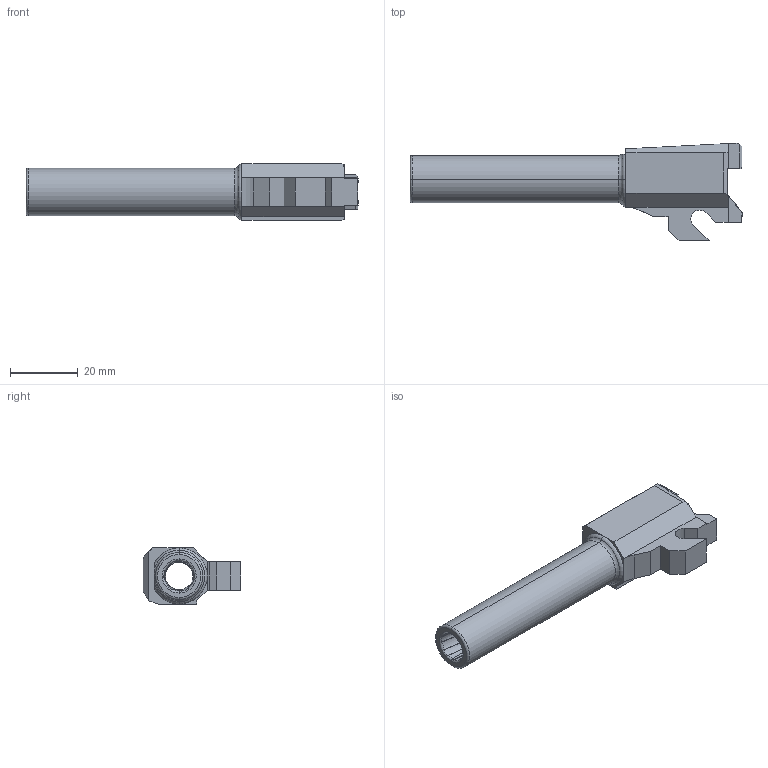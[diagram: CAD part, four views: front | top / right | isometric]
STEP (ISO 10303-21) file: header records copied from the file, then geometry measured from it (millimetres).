
FILE_DESCRIPTION (( 'STEP AP214' ), '1' );
FILE_NAME ('Barrel.step', '2014-07-30T19:45:38', ( 'WarFairy' ), ( '' ), 'SwSTEP 2.0', 'SolidWorks 2013', '' );
FILE_SCHEMA (( 'AUTOMOTIVE_DESIGN' ));
Length unit declared in the file: millimetre
Products named in the file (1): Barrel
Bounding box: 98.09 x 28.93 x 16.68 mm (x, y, z)
Volume: 13429 mm3; surface area: 8519.6 mm2
Topology: 1 solids, 1 shells, 276 faces, 761 edges, 501 vertices
Faces by surface type: plane 153, bspline 88, cylinder 20, torus 12, cone 3
Entity records: 10846 total; most frequent: CARTESIAN_POINT 4301, ORIENTED_EDGE 1522, DIRECTION 991, EDGE_CURVE 761, VERTEX_POINT 501, LINE 489, VECTOR 489, EDGE_LOOP 292
